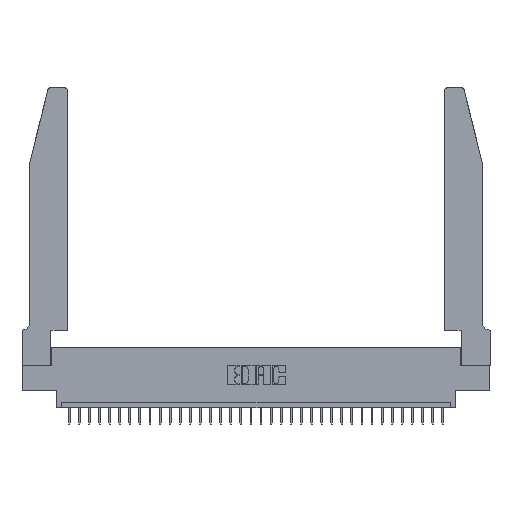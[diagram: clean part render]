
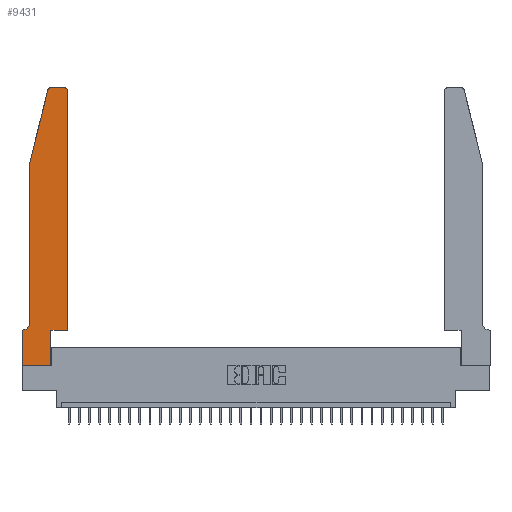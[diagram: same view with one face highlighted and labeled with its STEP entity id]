
A CAD part, top view. The second image highlights one B-rep face of the part: STEP entity #9431.
In plain terms, the highlighted planar face has unit normal (0, 0, 1).
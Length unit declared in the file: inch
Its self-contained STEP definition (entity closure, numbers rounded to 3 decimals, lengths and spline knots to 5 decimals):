
#63 = LINE ( 'NONE', #21123, #18653 ) ;
#82 = VERTEX_POINT ( 'NONE', #22660 ) ;
#109 = CARTESIAN_POINT ( 'NONE',  ( 0.4505, 0.35, 0.37 ) ) ;
#448 = EDGE_CURVE ( 'NONE', #2260, #28729, #11163, .T. ) ;
#608 = CARTESIAN_POINT ( 'NONE',  ( 0.4205, 2.72, 0.37 ) ) ;
#895 = CARTESIAN_POINT ( 'NONE',  ( 0.284, 2.75, 0.37 ) ) ;
#900 = CARTESIAN_POINT ( 'NONE',  ( 0.0755, 2., 0.37 ) ) ;
#1305 = AXIS2_PLACEMENT_3D ( 'NONE', #10206, #1811, #12493 ) ;
#1384 = LINE ( 'NONE', #28929, #23243 ) ;
#1751 = DIRECTION ( 'NONE',  ( -1., 0., 0. ) ) ;
#1811 = DIRECTION ( 'NONE',  ( 0., 0., 1. ) ) ;
#2036 = CARTESIAN_POINT ( 'NONE',  ( 0.2865, 0., 0.37 ) ) ;
#2260 = VERTEX_POINT ( 'NONE', #5607 ) ;
#3364 = ORIENTED_EDGE ( 'NONE', *, *, #448, .T. ) ;
#3365 = CARTESIAN_POINT ( 'NONE',  ( 0.4505, 0.35, 0.37 ) ) ;
#3567 = DIRECTION ( 'NONE',  ( 0., -1., 0. ) ) ;
#3699 = LINE ( 'NONE', #9673, #21058 ) ;
#4162 = EDGE_CURVE ( 'NONE', #16893, #4247, #1384, .T. ) ;
#4247 = VERTEX_POINT ( 'NONE', #18420 ) ;
#4423 = VECTOR ( 'NONE', #3567, 39.37008 ) ;
#4994 = CARTESIAN_POINT ( 'NONE',  ( 0.4205, 2.75, 0.37 ) ) ;
#5399 = DIRECTION ( 'NONE',  ( 0., 1., 0. ) ) ;
#5467 = EDGE_CURVE ( 'NONE', #28729, #14361, #63, .T. ) ;
#5607 = CARTESIAN_POINT ( 'NONE',  ( 0.4505, 2.72, 0.37 ) ) ;
#6531 = VECTOR ( 'NONE', #18986, 39.37008 ) ;
#6872 = CARTESIAN_POINT ( 'NONE',  ( 0.4505, 0.35, 0.37 ) ) ;
#7239 = CARTESIAN_POINT ( 'NONE',  ( 0., 0., 0.37 ) ) ;
#7487 = DIRECTION ( 'NONE',  ( 1., 0., 0. ) ) ;
#7718 = ORIENTED_EDGE ( 'NONE', *, *, #24672, .T. ) ;
#7727 = CIRCLE ( 'NONE', #29079, 0.07 ) ;
#8393 = VERTEX_POINT ( 'NONE', #26286 ) ;
#8642 = ORIENTED_EDGE ( 'NONE', *, *, #26624, .T. ) ;
#8799 = EDGE_CURVE ( 'NONE', #82, #8393, #7727, .T. ) ;
#9239 = ORIENTED_EDGE ( 'NONE', *, *, #33567, .T. ) ;
#9431 = ADVANCED_FACE ( 'NONE', ( #14327 ), #12847, .T. ) ;
#9673 = CARTESIAN_POINT ( 'NONE',  ( 0.0755, 0.35, 0.37 ) ) ;
#9962 = VERTEX_POINT ( 'NONE', #25037 ) ;
#10206 = CARTESIAN_POINT ( 'NONE',  ( 0., 0.35, 0.37 ) ) ;
#10661 = LINE ( 'NONE', #900, #4423 ) ;
#11163 = CIRCLE ( 'NONE', #11367, 0.03 ) ;
#11222 = CARTESIAN_POINT ( 'NONE',  ( 0., 0., 0.37 ) ) ;
#11367 = AXIS2_PLACEMENT_3D ( 'NONE', #608, #19215, #21593 ) ;
#11778 = EDGE_CURVE ( 'NONE', #30611, #2260, #31610, .T. ) ;
#12062 = DIRECTION ( 'NONE',  ( 1., 0., 0. ) ) ;
#12493 = DIRECTION ( 'NONE',  ( 1., 0., 0. ) ) ;
#12847 = PLANE ( 'NONE',  #1305 ) ;
#13401 = DIRECTION ( 'NONE',  ( -1., 0., 0. ) ) ;
#13438 = LINE ( 'NONE', #20211, #15109 ) ;
#13498 = CIRCLE ( 'NONE', #25261, 0.03 ) ;
#13697 = DIRECTION ( 'NONE',  ( -1., 0., 0. ) ) ;
#14259 = ORIENTED_EDGE ( 'NONE', *, *, #22681, .T. ) ;
#14327 = FACE_OUTER_BOUND ( 'NONE', #14466, .T. ) ;
#14361 = VERTEX_POINT ( 'NONE', #895 ) ;
#14435 = VECTOR ( 'NONE', #7487, 39.37008 ) ;
#14466 = EDGE_LOOP ( 'NONE', ( #29659, #29932, #7718, #14259, #19214, #19579, #9239, #8642, #14938, #15927, #29799, #3364 ) ) ;
#14882 = LINE ( 'NONE', #7239, #14435 ) ;
#14938 = ORIENTED_EDGE ( 'NONE', *, *, #4162, .T. ) ;
#15085 = VERTEX_POINT ( 'NONE', #22611 ) ;
#15109 = VECTOR ( 'NONE', #25571, 39.37008 ) ;
#15685 = DIRECTION ( 'NONE',  ( 0., 0., 1. ) ) ;
#15927 = ORIENTED_EDGE ( 'NONE', *, *, #28464, .T. ) ;
#16893 = VERTEX_POINT ( 'NONE', #2036 ) ;
#18324 = DIRECTION ( 'NONE',  ( 1., 0., 0. ) ) ;
#18420 = CARTESIAN_POINT ( 'NONE',  ( 0.2865, 0.35, 0.37 ) ) ;
#18653 = VECTOR ( 'NONE', #13401, 39.37008 ) ;
#18889 = CARTESIAN_POINT ( 'NONE',  ( 0.0055, 0.42, 0.37 ) ) ;
#18891 = CARTESIAN_POINT ( 'NONE',  ( 0.284, 2.72, 0.37 ) ) ;
#18986 = DIRECTION ( 'NONE',  ( 0., 1., 0. ) ) ;
#19214 = ORIENTED_EDGE ( 'NONE', *, *, #8799, .T. ) ;
#19215 = DIRECTION ( 'NONE',  ( 0., 0., 1. ) ) ;
#19464 = DIRECTION ( 'NONE',  ( -0.239, -0.971, 0. ) ) ;
#19579 = ORIENTED_EDGE ( 'NONE', *, *, #26577, .T. ) ;
#20211 = CARTESIAN_POINT ( 'NONE',  ( 0., 0., 0.37 ) ) ;
#20349 = VECTOR ( 'NONE', #19464, 39.37008 ) ;
#21058 = VECTOR ( 'NONE', #1751, 39.37008 ) ;
#21123 = CARTESIAN_POINT ( 'NONE',  ( 0.2605, 2.75, 0.37 ) ) ;
#21157 = LINE ( 'NONE', #22390, #20349 ) ;
#21497 = DIRECTION ( 'NONE',  ( 0., 0., -1. ) ) ;
#21593 = DIRECTION ( 'NONE',  ( 1., 0., 0. ) ) ;
#22390 = CARTESIAN_POINT ( 'NONE',  ( 0.0755, 2., 0.37 ) ) ;
#22578 = VECTOR ( 'NONE', #12062, 39.37008 ) ;
#22611 = CARTESIAN_POINT ( 'NONE',  ( 0., 0.35, 0.37 ) ) ;
#22660 = CARTESIAN_POINT ( 'NONE',  ( 0.0755, 0.42, 0.37 ) ) ;
#22681 = EDGE_CURVE ( 'NONE', #32653, #82, #10661, .T. ) ;
#22834 = EDGE_CURVE ( 'NONE', #14361, #9962, #13498, .T. ) ;
#23243 = VECTOR ( 'NONE', #5399, 39.37008 ) ;
#24672 = EDGE_CURVE ( 'NONE', #9962, #32653, #21157, .T. ) ;
#25037 = CARTESIAN_POINT ( 'NONE',  ( 0.25487, 2.72718, 0.37 ) ) ;
#25261 = AXIS2_PLACEMENT_3D ( 'NONE', #18891, #15685, #18324 ) ;
#25571 = DIRECTION ( 'NONE',  ( 0., -1., 0. ) ) ;
#26286 = CARTESIAN_POINT ( 'NONE',  ( 0.0055, 0.35, 0.37 ) ) ;
#26577 = EDGE_CURVE ( 'NONE', #8393, #15085, #3699, .T. ) ;
#26624 = EDGE_CURVE ( 'NONE', #31185, #16893, #14882, .T. ) ;
#28464 = EDGE_CURVE ( 'NONE', #4247, #30611, #29543, .T. ) ;
#28729 = VERTEX_POINT ( 'NONE', #4994 ) ;
#28929 = CARTESIAN_POINT ( 'NONE',  ( 0.2865, 0.35, 0.37 ) ) ;
#29079 = AXIS2_PLACEMENT_3D ( 'NONE', #18889, #21497, #13697 ) ;
#29543 = LINE ( 'NONE', #6872, #22578 ) ;
#29659 = ORIENTED_EDGE ( 'NONE', *, *, #5467, .T. ) ;
#29799 = ORIENTED_EDGE ( 'NONE', *, *, #11778, .T. ) ;
#29932 = ORIENTED_EDGE ( 'NONE', *, *, #22834, .T. ) ;
#30611 = VERTEX_POINT ( 'NONE', #109 ) ;
#31185 = VERTEX_POINT ( 'NONE', #11222 ) ;
#31610 = LINE ( 'NONE', #3365, #6531 ) ;
#32653 = VERTEX_POINT ( 'NONE', #33738 ) ;
#33567 = EDGE_CURVE ( 'NONE', #15085, #31185, #13438, .T. ) ;
#33738 = CARTESIAN_POINT ( 'NONE',  ( 0.0755, 2., 0.37 ) ) ;
